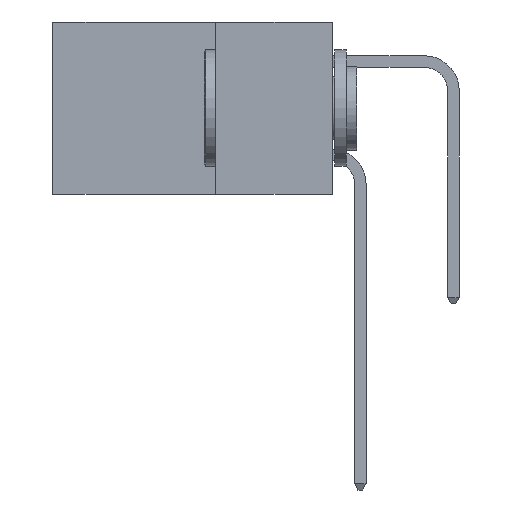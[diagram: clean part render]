
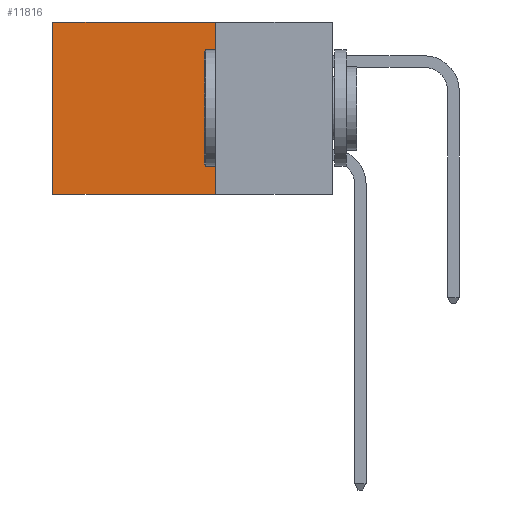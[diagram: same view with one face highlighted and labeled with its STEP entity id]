
A CAD part, left-side view. The second image highlights one B-rep face of the part: STEP entity #11816.
In plain terms, the highlighted planar face has unit normal (-1, 0, 0).
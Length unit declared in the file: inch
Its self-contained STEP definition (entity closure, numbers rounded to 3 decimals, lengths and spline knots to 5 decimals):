
#583 = DIRECTION ( 'NONE',  ( 0., 0., -1. ) ) ;
#1406 = ORIENTED_EDGE ( 'NONE', *, *, #7885, .T. ) ;
#1824 = VECTOR ( 'NONE', #17988, 39.37008 ) ;
#2357 = ORIENTED_EDGE ( 'NONE', *, *, #20927, .F. ) ;
#2822 = ORIENTED_EDGE ( 'NONE', *, *, #13756, .F. ) ;
#3816 = EDGE_LOOP ( 'NONE', ( #20986, #2357, #2822, #1406 ) ) ;
#3832 = VERTEX_POINT ( 'NONE', #17708 ) ;
#3854 = CARTESIAN_POINT ( 'NONE',  ( 0.2615, 0.25, -0.37 ) ) ;
#4180 = CARTESIAN_POINT ( 'NONE',  ( 0.2615, 0.25, -0.37 ) ) ;
#5000 = DIRECTION ( 'NONE',  ( 0., 1., 0. ) ) ;
#5599 = DIRECTION ( 'NONE',  ( 0., 0., -1. ) ) ;
#7051 = LINE ( 'NONE', #4180, #1824 ) ;
#7351 = CARTESIAN_POINT ( 'NONE',  ( 0.2615, 0.6, -0.37 ) ) ;
#7373 = LINE ( 'NONE', #20469, #11448 ) ;
#7403 = VERTEX_POINT ( 'NONE', #18054 ) ;
#7885 = EDGE_CURVE ( 'NONE', #3832, #7403, #18600, .T. ) ;
#8649 = EDGE_CURVE ( 'NONE', #7403, #12935, #13257, .T. ) ;
#9283 = CARTESIAN_POINT ( 'NONE',  ( 0.2615, 0.25, 0. ) ) ;
#10050 = VECTOR ( 'NONE', #11011, 39.37008 ) ;
#11011 = DIRECTION ( 'NONE',  ( 0., 1., 0. ) ) ;
#11448 = VECTOR ( 'NONE', #5000, 39.37008 ) ;
#11816 = ADVANCED_FACE ( 'NONE', ( #17939 ), #14253, .F. ) ;
#12724 = VECTOR ( 'NONE', #583, 39.37008 ) ;
#12935 = VERTEX_POINT ( 'NONE', #7351 ) ;
#13257 = LINE ( 'NONE', #19626, #12724 ) ;
#13756 = EDGE_CURVE ( 'NONE', #3832, #14883, #7051, .T. ) ;
#14253 = PLANE ( 'NONE',  #19569 ) ;
#14883 = VERTEX_POINT ( 'NONE', #16023 ) ;
#15964 = DIRECTION ( 'NONE',  ( 1., 0., 0. ) ) ;
#16023 = CARTESIAN_POINT ( 'NONE',  ( 0.2615, 0.25, -0.37 ) ) ;
#17708 = CARTESIAN_POINT ( 'NONE',  ( 0.2615, 0.25, 0. ) ) ;
#17939 = FACE_OUTER_BOUND ( 'NONE', #3816, .T. ) ;
#17988 = DIRECTION ( 'NONE',  ( 0., 0., -1. ) ) ;
#18054 = CARTESIAN_POINT ( 'NONE',  ( 0.2615, 0.6, 0. ) ) ;
#18600 = LINE ( 'NONE', #9283, #10050 ) ;
#19569 = AXIS2_PLACEMENT_3D ( 'NONE', #3854, #15964, #5599 ) ;
#19626 = CARTESIAN_POINT ( 'NONE',  ( 0.2615, 0.6, -0.37 ) ) ;
#20469 = CARTESIAN_POINT ( 'NONE',  ( 0.2615, 0.25, -0.37 ) ) ;
#20927 = EDGE_CURVE ( 'NONE', #14883, #12935, #7373, .T. ) ;
#20986 = ORIENTED_EDGE ( 'NONE', *, *, #8649, .T. ) ;
